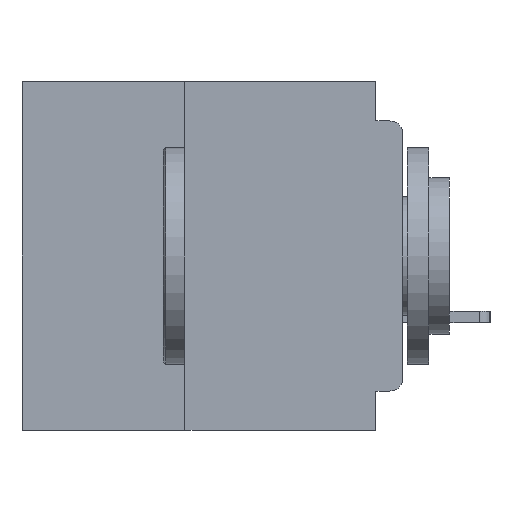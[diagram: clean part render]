
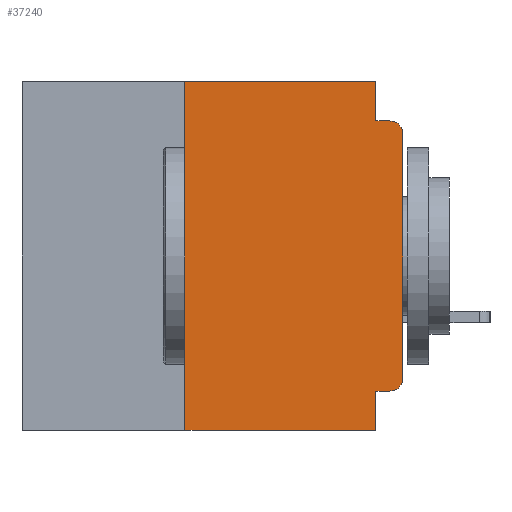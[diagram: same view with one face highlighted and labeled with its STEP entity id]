
A CAD part, left-side view. The second image highlights one B-rep face of the part: STEP entity #37240.
In plain terms, the highlighted planar face has unit normal (-1, 0, 0).
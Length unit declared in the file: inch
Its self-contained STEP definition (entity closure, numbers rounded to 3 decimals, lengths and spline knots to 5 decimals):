
#338 = ORIENTED_EDGE ( 'NONE', *, *, #35071, .F. ) ;
#1475 = PLANE ( 'NONE',  #14948 ) ;
#1911 = LINE ( 'NONE', #25829, #8858 ) ;
#2224 = ORIENTED_EDGE ( 'NONE', *, *, #37791, .F. ) ;
#3007 = CARTESIAN_POINT ( 'NONE',  ( 0., 0.437, -0.4 ) ) ;
#3739 = CARTESIAN_POINT ( 'NONE',  ( 0., 0.25, -0.4 ) ) ;
#4517 = ORIENTED_EDGE ( 'NONE', *, *, #19193, .F. ) ;
#4909 = VERTEX_POINT ( 'NONE', #30475 ) ;
#5377 = VECTOR ( 'NONE', #16361, 39.37008 ) ;
#5477 = EDGE_CURVE ( 'NONE', #31927, #6027, #15810, .T. ) ;
#6021 = DIRECTION ( 'NONE',  ( 0., -1., 0. ) ) ;
#6027 = VERTEX_POINT ( 'NONE', #24430 ) ;
#6101 = VECTOR ( 'NONE', #6021, 39.37008 ) ;
#6434 = EDGE_CURVE ( 'NONE', #4909, #15969, #33544, .T. ) ;
#6722 = DIRECTION ( 'NONE',  ( 0., 0., 1. ) ) ;
#7182 = CARTESIAN_POINT ( 'NONE',  ( 0., 0.015, -0.06 ) ) ;
#7912 = LINE ( 'NONE', #18621, #21687 ) ;
#8858 = VECTOR ( 'NONE', #17095, 39.37008 ) ;
#9157 = ORIENTED_EDGE ( 'NONE', *, *, #20212, .F. ) ;
#9431 = CARTESIAN_POINT ( 'NONE',  ( 0., 0., -0.34 ) ) ;
#9619 = ORIENTED_EDGE ( 'NONE', *, *, #20841, .T. ) ;
#10141 = DIRECTION ( 'NONE',  ( 0., 0., -1. ) ) ;
#11320 = EDGE_CURVE ( 'NONE', #15969, #37313, #20378, .T. ) ;
#11480 = ORIENTED_EDGE ( 'NONE', *, *, #11818, .T. ) ;
#11818 = EDGE_CURVE ( 'NONE', #31927, #13653, #23595, .T. ) ;
#11845 = LINE ( 'NONE', #29670, #26524 ) ;
#13153 = VECTOR ( 'NONE', #13823, 39.37008 ) ;
#13653 = VERTEX_POINT ( 'NONE', #35857 ) ;
#13823 = DIRECTION ( 'NONE',  ( 0., -1., 0. ) ) ;
#14358 = VERTEX_POINT ( 'NONE', #16266 ) ;
#14610 = DIRECTION ( 'NONE',  ( -1., 0., 0. ) ) ;
#14767 = CARTESIAN_POINT ( 'NONE',  ( 0., 0., 0. ) ) ;
#14948 = AXIS2_PLACEMENT_3D ( 'NONE', #36483, #33809, #16310 ) ;
#15050 = DIRECTION ( 'NONE',  ( 0., -1., 0. ) ) ;
#15154 = ORIENTED_EDGE ( 'NONE', *, *, #35387, .F. ) ;
#15810 = LINE ( 'NONE', #3739, #29536 ) ;
#15969 = VERTEX_POINT ( 'NONE', #9431 ) ;
#16266 = CARTESIAN_POINT ( 'NONE',  ( 0., 0.031, 0. ) ) ;
#16310 = DIRECTION ( 'NONE',  ( 0., 0., -1. ) ) ;
#16361 = DIRECTION ( 'NONE',  ( 0., 1., 0. ) ) ;
#17095 = DIRECTION ( 'NONE',  ( 0., 0., -1. ) ) ;
#17895 = ORIENTED_EDGE ( 'NONE', *, *, #6434, .T. ) ;
#18335 = VERTEX_POINT ( 'NONE', #30853 ) ;
#18621 = CARTESIAN_POINT ( 'NONE',  ( 0., 0.031, -0.4 ) ) ;
#18737 = DIRECTION ( 'NONE',  ( 0., 0., -1. ) ) ;
#19193 = EDGE_CURVE ( 'NONE', #21293, #31817, #11845, .T. ) ;
#20212 = EDGE_CURVE ( 'NONE', #6027, #14358, #37360, .T. ) ;
#20378 = LINE ( 'NONE', #14767, #36818 ) ;
#20841 = EDGE_CURVE ( 'NONE', #37313, #31817, #21355, .T. ) ;
#21026 = LINE ( 'NONE', #33744, #5377 ) ;
#21293 = VERTEX_POINT ( 'NONE', #26773 ) ;
#21355 = CIRCLE ( 'NONE', #21548, 0.015 ) ;
#21548 = AXIS2_PLACEMENT_3D ( 'NONE', #7182, #27711, #10141 ) ;
#21687 = VECTOR ( 'NONE', #18737, 39.37008 ) ;
#23595 = LINE ( 'NONE', #3007, #6101 ) ;
#23667 = CARTESIAN_POINT ( 'NONE',  ( 0., 0.015, -0.045 ) ) ;
#24430 = CARTESIAN_POINT ( 'NONE',  ( 0., 0.25, 0. ) ) ;
#25829 = CARTESIAN_POINT ( 'NONE',  ( 0., 0.031, 0. ) ) ;
#26524 = VECTOR ( 'NONE', #15050, 39.37008 ) ;
#26564 = FACE_OUTER_BOUND ( 'NONE', #27589, .T. ) ;
#26773 = CARTESIAN_POINT ( 'NONE',  ( 0., 0.031, -0.045 ) ) ;
#27237 = CARTESIAN_POINT ( 'NONE',  ( 0., 0.25, -0.4 ) ) ;
#27589 = EDGE_LOOP ( 'NONE', ( #37021, #9619, #4517, #338, #9157, #32082, #11480, #15154, #2224, #17895 ) ) ;
#27711 = DIRECTION ( 'NONE',  ( -1., 0., 0. ) ) ;
#28351 = CARTESIAN_POINT ( 'NONE',  ( 0., 0., -0.06 ) ) ;
#29536 = VECTOR ( 'NONE', #6722, 39.37008 ) ;
#29670 = CARTESIAN_POINT ( 'NONE',  ( 0., 0., -0.045 ) ) ;
#30475 = CARTESIAN_POINT ( 'NONE',  ( 0., 0.015, -0.355 ) ) ;
#30853 = CARTESIAN_POINT ( 'NONE',  ( 0., 0.031, -0.355 ) ) ;
#31817 = VERTEX_POINT ( 'NONE', #23667 ) ;
#31927 = VERTEX_POINT ( 'NONE', #27237 ) ;
#32082 = ORIENTED_EDGE ( 'NONE', *, *, #5477, .F. ) ;
#32165 = CARTESIAN_POINT ( 'NONE',  ( 0., 0.015, -0.34 ) ) ;
#33544 = CIRCLE ( 'NONE', #36821, 0.015 ) ;
#33744 = CARTESIAN_POINT ( 'NONE',  ( 0., 0., -0.355 ) ) ;
#33809 = DIRECTION ( 'NONE',  ( 1., 0., 0. ) ) ;
#34272 = CARTESIAN_POINT ( 'NONE',  ( 0., 0.437, 0. ) ) ;
#35061 = DIRECTION ( 'NONE',  ( 0., 0., -1. ) ) ;
#35071 = EDGE_CURVE ( 'NONE', #14358, #21293, #1911, .T. ) ;
#35222 = DIRECTION ( 'NONE',  ( 0., 0., 1. ) ) ;
#35387 = EDGE_CURVE ( 'NONE', #18335, #13653, #7912, .T. ) ;
#35857 = CARTESIAN_POINT ( 'NONE',  ( 0., 0.031, -0.4 ) ) ;
#36483 = CARTESIAN_POINT ( 'NONE',  ( 0., 0.437, 0. ) ) ;
#36818 = VECTOR ( 'NONE', #35222, 39.37008 ) ;
#36821 = AXIS2_PLACEMENT_3D ( 'NONE', #32165, #14610, #35061 ) ;
#37021 = ORIENTED_EDGE ( 'NONE', *, *, #11320, .T. ) ;
#37240 = ADVANCED_FACE ( 'NONE', ( #26564 ), #1475, .F. ) ;
#37313 = VERTEX_POINT ( 'NONE', #28351 ) ;
#37360 = LINE ( 'NONE', #34272, #13153 ) ;
#37791 = EDGE_CURVE ( 'NONE', #4909, #18335, #21026, .T. ) ;
